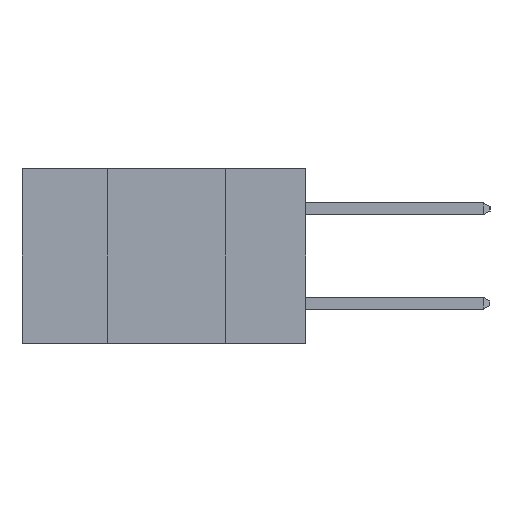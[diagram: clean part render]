
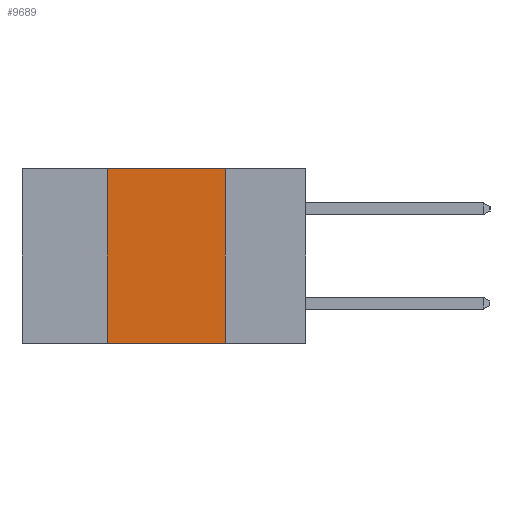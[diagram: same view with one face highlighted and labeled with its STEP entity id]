
A CAD part, left-side view. The second image highlights one B-rep face of the part: STEP entity #9689.
In plain terms, the highlighted planar face has unit normal (-1, 0, 0).
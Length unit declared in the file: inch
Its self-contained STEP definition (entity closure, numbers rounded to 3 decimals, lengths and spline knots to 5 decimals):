
#689 = VECTOR ( 'NONE', #5195, 39.37008 ) ;
#1253 = FACE_OUTER_BOUND ( 'NONE', #9948, .T. ) ;
#1774 = ORIENTED_EDGE ( 'NONE', *, *, #1864, .F. ) ;
#1864 = EDGE_CURVE ( 'NONE', #11573, #11792, #10901, .T. ) ;
#2126 = EDGE_CURVE ( 'NONE', #11792, #8925, #10083, .T. ) ;
#2681 = DIRECTION ( 'NONE',  ( 0., -1., 0. ) ) ;
#3279 = ORIENTED_EDGE ( 'NONE', *, *, #2126, .F. ) ;
#3829 = ORIENTED_EDGE ( 'NONE', *, *, #4055, .T. ) ;
#4055 = EDGE_CURVE ( 'NONE', #11573, #5297, #14227, .T. ) ;
#4881 = CARTESIAN_POINT ( 'NONE',  ( 0., 0.42, 0. ) ) ;
#5195 = DIRECTION ( 'NONE',  ( 0., 0., -1. ) ) ;
#5297 = VERTEX_POINT ( 'NONE', #10242 ) ;
#5312 = CARTESIAN_POINT ( 'NONE',  ( 0., 0.6, -0.37 ) ) ;
#5762 = VECTOR ( 'NONE', #5797, 39.37008 ) ;
#5797 = DIRECTION ( 'NONE',  ( 0., -1., 0. ) ) ;
#6426 = DIRECTION ( 'NONE',  ( 0., 0., -1. ) ) ;
#6695 = CARTESIAN_POINT ( 'NONE',  ( 0., 0.42, -0.37 ) ) ;
#6920 = LINE ( 'NONE', #8603, #689 ) ;
#7064 = VECTOR ( 'NONE', #2681, 39.37008 ) ;
#7311 = CARTESIAN_POINT ( 'NONE',  ( 0., 0.42, 0. ) ) ;
#7430 = DIRECTION ( 'NONE',  ( 0., 0., 1. ) ) ;
#7551 = CARTESIAN_POINT ( 'NONE',  ( 0., 0.6, 0. ) ) ;
#8362 = EDGE_CURVE ( 'NONE', #8925, #5297, #6920, .T. ) ;
#8603 = CARTESIAN_POINT ( 'NONE',  ( 0., 0.17, 0. ) ) ;
#8925 = VERTEX_POINT ( 'NONE', #10533 ) ;
#9689 = ADVANCED_FACE ( 'NONE', ( #1253 ), #11956, .F. ) ;
#9948 = EDGE_LOOP ( 'NONE', ( #11944, #3279, #1774, #3829 ) ) ;
#10083 = LINE ( 'NONE', #11331, #7064 ) ;
#10242 = CARTESIAN_POINT ( 'NONE',  ( 0., 0.17, -0.37 ) ) ;
#10533 = CARTESIAN_POINT ( 'NONE',  ( 0., 0.17, 0. ) ) ;
#10570 = VECTOR ( 'NONE', #7430, 39.37008 ) ;
#10901 = LINE ( 'NONE', #7311, #10570 ) ;
#11331 = CARTESIAN_POINT ( 'NONE',  ( 0., 0.6, 0. ) ) ;
#11573 = VERTEX_POINT ( 'NONE', #6695 ) ;
#11792 = VERTEX_POINT ( 'NONE', #4881 ) ;
#11944 = ORIENTED_EDGE ( 'NONE', *, *, #8362, .F. ) ;
#11956 = PLANE ( 'NONE',  #12751 ) ;
#12751 = AXIS2_PLACEMENT_3D ( 'NONE', #7551, #13081, #6426 ) ;
#13081 = DIRECTION ( 'NONE',  ( 1., 0., 0. ) ) ;
#14227 = LINE ( 'NONE', #5312, #5762 ) ;
